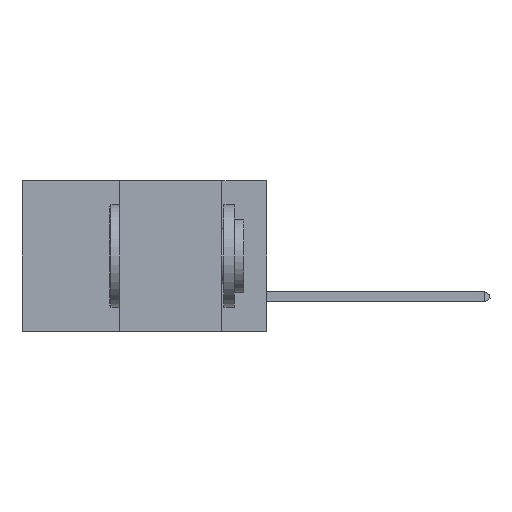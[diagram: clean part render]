
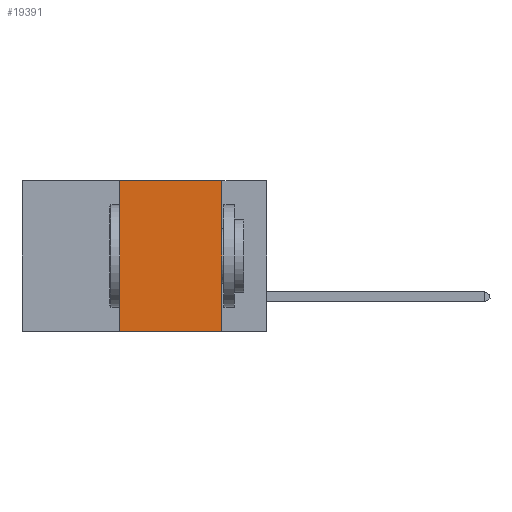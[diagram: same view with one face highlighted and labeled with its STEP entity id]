
A CAD part, left-side view. The second image highlights one B-rep face of the part: STEP entity #19391.
In plain terms, the highlighted planar face has unit normal (-1, 0, 0).
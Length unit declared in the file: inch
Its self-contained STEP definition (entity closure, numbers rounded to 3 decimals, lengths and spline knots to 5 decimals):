
#83 = LINE ( 'NONE', #29889, #28662 ) ;
#1330 = CARTESIAN_POINT ( 'NONE',  ( 0., 0.36, -0.37 ) ) ;
#1598 = LINE ( 'NONE', #1869, #19969 ) ;
#1869 = CARTESIAN_POINT ( 'NONE',  ( 0., 0.36, 0. ) ) ;
#3443 = ORIENTED_EDGE ( 'NONE', *, *, #16872, .F. ) ;
#3743 = DIRECTION ( 'NONE',  ( 1., 0., 0. ) ) ;
#4635 = EDGE_CURVE ( 'NONE', #5344, #12453, #18312, .T. ) ;
#5307 = AXIS2_PLACEMENT_3D ( 'NONE', #17443, #3743, #19800 ) ;
#5344 = VERTEX_POINT ( 'NONE', #1330 ) ;
#6824 = VECTOR ( 'NONE', #10238, 39.37008 ) ;
#8209 = FACE_OUTER_BOUND ( 'NONE', #23196, .T. ) ;
#8804 = VERTEX_POINT ( 'NONE', #11560 ) ;
#10005 = EDGE_CURVE ( 'NONE', #17139, #8804, #83, .T. ) ;
#10238 = DIRECTION ( 'NONE',  ( 0., -1., 0. ) ) ;
#11560 = CARTESIAN_POINT ( 'NONE',  ( 0., 0.11, 0. ) ) ;
#11919 = CARTESIAN_POINT ( 'NONE',  ( 0., 0.11, 0. ) ) ;
#12453 = VERTEX_POINT ( 'NONE', #20130 ) ;
#13389 = VECTOR ( 'NONE', #16532, 39.37008 ) ;
#15330 = EDGE_CURVE ( 'NONE', #5344, #17139, #1598, .T. ) ;
#16532 = DIRECTION ( 'NONE',  ( 0., 0., -1. ) ) ;
#16872 = EDGE_CURVE ( 'NONE', #8804, #12453, #18820, .T. ) ;
#17139 = VERTEX_POINT ( 'NONE', #17849 ) ;
#17443 = CARTESIAN_POINT ( 'NONE',  ( 0., 0.6, 0. ) ) ;
#17849 = CARTESIAN_POINT ( 'NONE',  ( 0., 0.36, 0. ) ) ;
#17939 = DIRECTION ( 'NONE',  ( 0., 0., 1. ) ) ;
#18312 = LINE ( 'NONE', #24093, #6824 ) ;
#18820 = LINE ( 'NONE', #11919, #13389 ) ;
#19391 = ADVANCED_FACE ( 'NONE', ( #8209 ), #26722, .F. ) ;
#19800 = DIRECTION ( 'NONE',  ( 0., 0., -1. ) ) ;
#19969 = VECTOR ( 'NONE', #17939, 39.37008 ) ;
#20130 = CARTESIAN_POINT ( 'NONE',  ( 0., 0.11, -0.37 ) ) ;
#22523 = ORIENTED_EDGE ( 'NONE', *, *, #10005, .F. ) ;
#22916 = DIRECTION ( 'NONE',  ( 0., -1., 0. ) ) ;
#23196 = EDGE_LOOP ( 'NONE', ( #3443, #22523, #28707, #23998 ) ) ;
#23998 = ORIENTED_EDGE ( 'NONE', *, *, #4635, .T. ) ;
#24093 = CARTESIAN_POINT ( 'NONE',  ( 0., 0.6, -0.37 ) ) ;
#26722 = PLANE ( 'NONE',  #5307 ) ;
#28662 = VECTOR ( 'NONE', #22916, 39.37008 ) ;
#28707 = ORIENTED_EDGE ( 'NONE', *, *, #15330, .F. ) ;
#29889 = CARTESIAN_POINT ( 'NONE',  ( 0., 0.6, 0. ) ) ;
